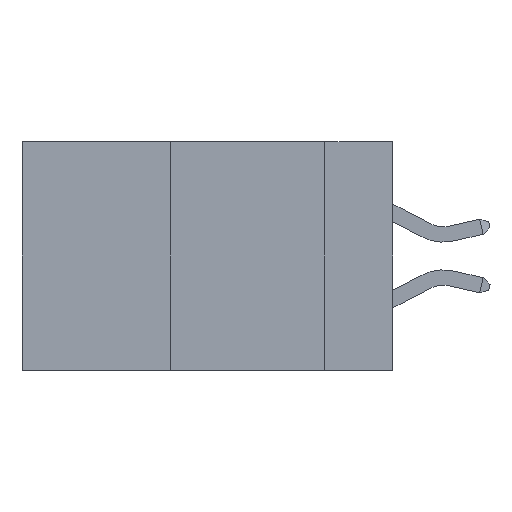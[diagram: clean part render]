
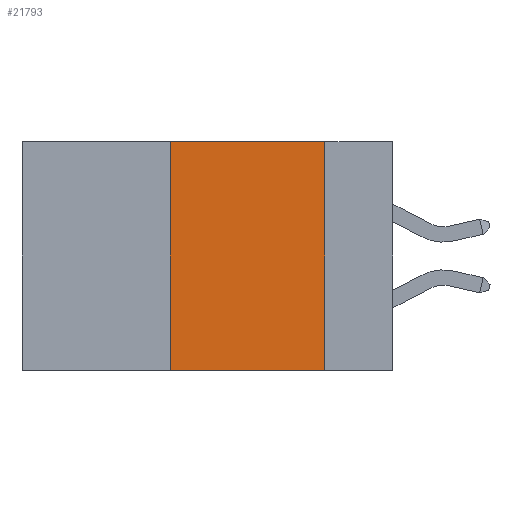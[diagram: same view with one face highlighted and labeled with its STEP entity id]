
A CAD part, left-side view. The second image highlights one B-rep face of the part: STEP entity #21793.
In plain terms, the highlighted planar face has unit normal (-1, 0, 0).
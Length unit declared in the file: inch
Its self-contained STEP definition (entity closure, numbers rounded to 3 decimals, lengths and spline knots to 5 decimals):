
#1211 = DIRECTION ( 'NONE',  ( 0., 0., 1. ) ) ;
#1346 = VERTEX_POINT ( 'NONE', #5098 ) ;
#1872 = DIRECTION ( 'NONE',  ( 0., 0., -1. ) ) ;
#2289 = PLANE ( 'NONE',  #18565 ) ;
#3416 = ORIENTED_EDGE ( 'NONE', *, *, #13283, .F. ) ;
#4079 = DIRECTION ( 'NONE',  ( 1., 0., 0. ) ) ;
#4963 = VERTEX_POINT ( 'NONE', #25241 ) ;
#5098 = CARTESIAN_POINT ( 'NONE',  ( 0., 0.11, -0.37 ) ) ;
#7000 = LINE ( 'NONE', #19569, #11870 ) ;
#7166 = CARTESIAN_POINT ( 'NONE',  ( 0., 0.36, -0.37 ) ) ;
#7497 = LINE ( 'NONE', #12176, #24714 ) ;
#8387 = CARTESIAN_POINT ( 'NONE',  ( 0., 0.6, 0. ) ) ;
#8672 = VECTOR ( 'NONE', #15467, 39.37008 ) ;
#9852 = EDGE_CURVE ( 'NONE', #16322, #1346, #7497, .T. ) ;
#10585 = DIRECTION ( 'NONE',  ( 0., 0., -1. ) ) ;
#11742 = CARTESIAN_POINT ( 'NONE',  ( 0., 0.11, 0. ) ) ;
#11870 = VECTOR ( 'NONE', #1211, 39.37008 ) ;
#12176 = CARTESIAN_POINT ( 'NONE',  ( 0., 0.11, 0. ) ) ;
#12493 = DIRECTION ( 'NONE',  ( 0., -1., 0. ) ) ;
#13283 = EDGE_CURVE ( 'NONE', #14605, #4963, #7000, .T. ) ;
#14383 = ORIENTED_EDGE ( 'NONE', *, *, #17130, .F. ) ;
#14573 = ORIENTED_EDGE ( 'NONE', *, *, #9852, .F. ) ;
#14605 = VERTEX_POINT ( 'NONE', #7166 ) ;
#15197 = CARTESIAN_POINT ( 'NONE',  ( 0., 0.6, -0.37 ) ) ;
#15467 = DIRECTION ( 'NONE',  ( 0., -1., 0. ) ) ;
#15849 = EDGE_LOOP ( 'NONE', ( #14573, #14383, #3416, #16373 ) ) ;
#16322 = VERTEX_POINT ( 'NONE', #11742 ) ;
#16373 = ORIENTED_EDGE ( 'NONE', *, *, #21942, .T. ) ;
#17130 = EDGE_CURVE ( 'NONE', #4963, #16322, #19964, .T. ) ;
#18565 = AXIS2_PLACEMENT_3D ( 'NONE', #22757, #4079, #10585 ) ;
#19569 = CARTESIAN_POINT ( 'NONE',  ( 0., 0.36, 0. ) ) ;
#19653 = VECTOR ( 'NONE', #12493, 39.37008 ) ;
#19964 = LINE ( 'NONE', #8387, #19653 ) ;
#21695 = LINE ( 'NONE', #15197, #8672 ) ;
#21793 = ADVANCED_FACE ( 'NONE', ( #22646 ), #2289, .F. ) ;
#21942 = EDGE_CURVE ( 'NONE', #14605, #1346, #21695, .T. ) ;
#22646 = FACE_OUTER_BOUND ( 'NONE', #15849, .T. ) ;
#22757 = CARTESIAN_POINT ( 'NONE',  ( 0., 0.6, 0. ) ) ;
#24714 = VECTOR ( 'NONE', #1872, 39.37008 ) ;
#25241 = CARTESIAN_POINT ( 'NONE',  ( 0., 0.36, 0. ) ) ;
